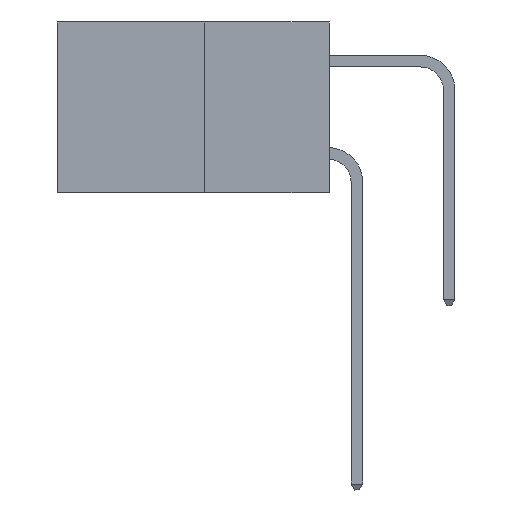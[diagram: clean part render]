
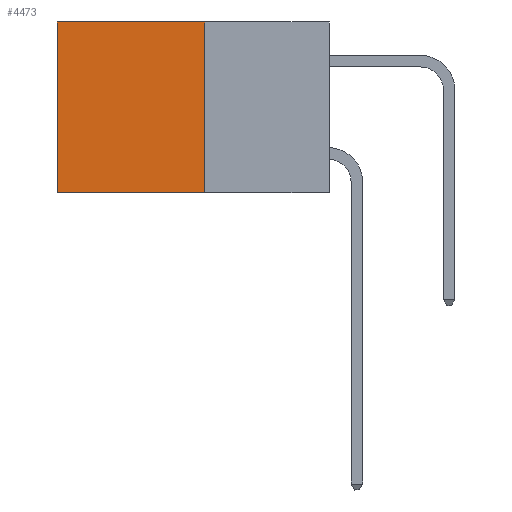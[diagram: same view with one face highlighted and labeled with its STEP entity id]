
A CAD part, left-side view. The second image highlights one B-rep face of the part: STEP entity #4473.
In plain terms, the highlighted planar face has unit normal (-1, 0, 0).
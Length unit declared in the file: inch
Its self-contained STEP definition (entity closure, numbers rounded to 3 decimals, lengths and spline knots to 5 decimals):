
#917 = CARTESIAN_POINT ( 'NONE',  ( 0.277, 0.27, -0.37 ) ) ;
#1149 = DIRECTION ( 'NONE',  ( 0., 0., -1. ) ) ;
#3559 = CARTESIAN_POINT ( 'NONE',  ( 0.277, 0.27, -0.37 ) ) ;
#3590 = ORIENTED_EDGE ( 'NONE', *, *, #18328, .F. ) ;
#4424 = VERTEX_POINT ( 'NONE', #12231 ) ;
#4473 = ADVANCED_FACE ( 'NONE', ( #14475 ), #26876, .F. ) ;
#5224 = ORIENTED_EDGE ( 'NONE', *, *, #10492, .T. ) ;
#5412 = CARTESIAN_POINT ( 'NONE',  ( 0.277, 0.59, -0.37 ) ) ;
#5522 = DIRECTION ( 'NONE',  ( 0., 1., 0. ) ) ;
#5538 = VERTEX_POINT ( 'NONE', #27649 ) ;
#5787 = CARTESIAN_POINT ( 'NONE',  ( 0.277, 0.27, -0.37 ) ) ;
#6013 = EDGE_CURVE ( 'NONE', #4424, #26474, #12249, .T. ) ;
#7191 = LINE ( 'NONE', #28410, #24496 ) ;
#8178 = LINE ( 'NONE', #917, #26073 ) ;
#8426 = DIRECTION ( 'NONE',  ( 0., 0., -1. ) ) ;
#10492 = EDGE_CURVE ( 'NONE', #5538, #27618, #7191, .T. ) ;
#10751 = DIRECTION ( 'NONE',  ( 1., 0., 0. ) ) ;
#11991 = CARTESIAN_POINT ( 'NONE',  ( 0.277, 0.27, 0. ) ) ;
#12231 = CARTESIAN_POINT ( 'NONE',  ( 0.277, 0.27, 0. ) ) ;
#12249 = LINE ( 'NONE', #17778, #18247 ) ;
#14034 = ORIENTED_EDGE ( 'NONE', *, *, #6013, .F. ) ;
#14247 = DIRECTION ( 'NONE',  ( 0., 1., 0. ) ) ;
#14475 = FACE_OUTER_BOUND ( 'NONE', #24025, .T. ) ;
#15446 = ORIENTED_EDGE ( 'NONE', *, *, #27693, .T. ) ;
#16122 = VECTOR ( 'NONE', #14247, 39.37008 ) ;
#17662 = DIRECTION ( 'NONE',  ( 0., 0., -1. ) ) ;
#17778 = CARTESIAN_POINT ( 'NONE',  ( 0.277, 0.27, -0.37 ) ) ;
#18247 = VECTOR ( 'NONE', #17662, 39.37008 ) ;
#18328 = EDGE_CURVE ( 'NONE', #26474, #27618, #8178, .T. ) ;
#24025 = EDGE_LOOP ( 'NONE', ( #5224, #3590, #14034, #15446 ) ) ;
#24496 = VECTOR ( 'NONE', #1149, 39.37008 ) ;
#26073 = VECTOR ( 'NONE', #5522, 39.37008 ) ;
#26474 = VERTEX_POINT ( 'NONE', #3559 ) ;
#26876 = PLANE ( 'NONE',  #28706 ) ;
#27618 = VERTEX_POINT ( 'NONE', #5412 ) ;
#27649 = CARTESIAN_POINT ( 'NONE',  ( 0.277, 0.59, 0. ) ) ;
#27693 = EDGE_CURVE ( 'NONE', #4424, #5538, #27749, .T. ) ;
#27749 = LINE ( 'NONE', #11991, #16122 ) ;
#28410 = CARTESIAN_POINT ( 'NONE',  ( 0.277, 0.59, -0.37 ) ) ;
#28706 = AXIS2_PLACEMENT_3D ( 'NONE', #5787, #10751, #8426 ) ;
